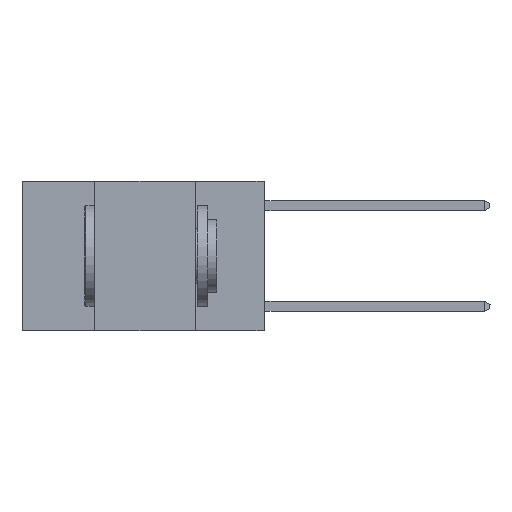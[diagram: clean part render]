
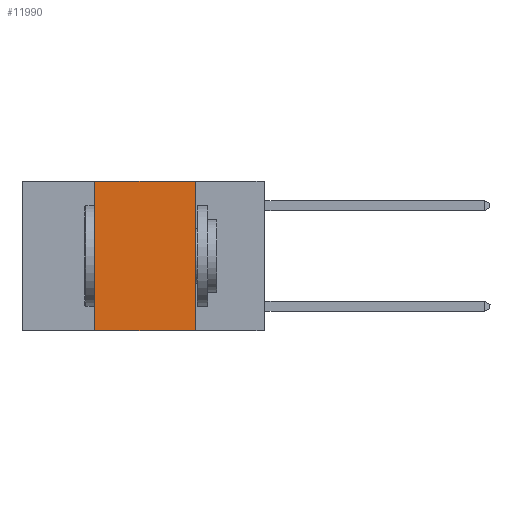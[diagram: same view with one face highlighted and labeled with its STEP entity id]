
A CAD part, left-side view. The second image highlights one B-rep face of the part: STEP entity #11990.
In plain terms, the highlighted planar face has unit normal (-1, 0, 0).
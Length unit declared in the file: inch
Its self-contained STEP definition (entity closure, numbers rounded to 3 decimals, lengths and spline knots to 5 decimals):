
#397 = DIRECTION ( 'NONE',  ( 0., 0., 1. ) ) ;
#681 = VERTEX_POINT ( 'NONE', #13861 ) ;
#860 = CARTESIAN_POINT ( 'NONE',  ( 0., 0.42, 0. ) ) ;
#1095 = VERTEX_POINT ( 'NONE', #26707 ) ;
#1295 = LINE ( 'NONE', #860, #12299 ) ;
#2452 = EDGE_CURVE ( 'NONE', #17114, #1095, #1295, .T. ) ;
#2572 = CARTESIAN_POINT ( 'NONE',  ( 0., 0.42, -0.37 ) ) ;
#2859 = DIRECTION ( 'NONE',  ( 1., 0., 0. ) ) ;
#3286 = ORIENTED_EDGE ( 'NONE', *, *, #5324, .F. ) ;
#3571 = LINE ( 'NONE', #7610, #20592 ) ;
#5324 = EDGE_CURVE ( 'NONE', #681, #17162, #10401, .T. ) ;
#6108 = VECTOR ( 'NONE', #17153, 39.37008 ) ;
#6495 = CARTESIAN_POINT ( 'NONE',  ( 0., 0.17, 0. ) ) ;
#7610 = CARTESIAN_POINT ( 'NONE',  ( 0., 0.6, -0.37 ) ) ;
#8727 = DIRECTION ( 'NONE',  ( 0., 0., -1. ) ) ;
#9068 = FACE_OUTER_BOUND ( 'NONE', #13479, .T. ) ;
#9220 = EDGE_CURVE ( 'NONE', #1095, #681, #23778, .T. ) ;
#9231 = AXIS2_PLACEMENT_3D ( 'NONE', #16087, #2859, #18367 ) ;
#9831 = DIRECTION ( 'NONE',  ( 0., -1., 0. ) ) ;
#10401 = LINE ( 'NONE', #6495, #21601 ) ;
#10471 = ORIENTED_EDGE ( 'NONE', *, *, #2452, .F. ) ;
#11990 = ADVANCED_FACE ( 'NONE', ( #9068 ), #24791, .F. ) ;
#12299 = VECTOR ( 'NONE', #397, 39.37008 ) ;
#13479 = EDGE_LOOP ( 'NONE', ( #3286, #20989, #10471, #27917 ) ) ;
#13861 = CARTESIAN_POINT ( 'NONE',  ( 0., 0.17, 0. ) ) ;
#16087 = CARTESIAN_POINT ( 'NONE',  ( 0., 0.6, 0. ) ) ;
#16316 = EDGE_CURVE ( 'NONE', #17114, #17162, #3571, .T. ) ;
#17114 = VERTEX_POINT ( 'NONE', #2572 ) ;
#17153 = DIRECTION ( 'NONE',  ( 0., -1., 0. ) ) ;
#17162 = VERTEX_POINT ( 'NONE', #18251 ) ;
#18251 = CARTESIAN_POINT ( 'NONE',  ( 0., 0.17, -0.37 ) ) ;
#18367 = DIRECTION ( 'NONE',  ( 0., 0., -1. ) ) ;
#20592 = VECTOR ( 'NONE', #9831, 39.37008 ) ;
#20989 = ORIENTED_EDGE ( 'NONE', *, *, #9220, .F. ) ;
#21601 = VECTOR ( 'NONE', #8727, 39.37008 ) ;
#23778 = LINE ( 'NONE', #25782, #6108 ) ;
#24791 = PLANE ( 'NONE',  #9231 ) ;
#25782 = CARTESIAN_POINT ( 'NONE',  ( 0., 0.6, 0. ) ) ;
#26707 = CARTESIAN_POINT ( 'NONE',  ( 0., 0.42, 0. ) ) ;
#27917 = ORIENTED_EDGE ( 'NONE', *, *, #16316, .T. ) ;
